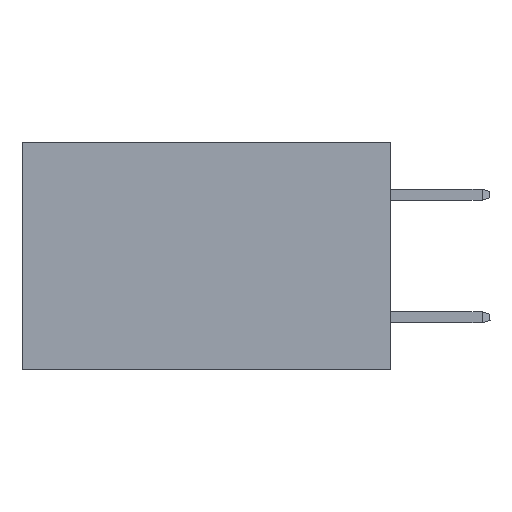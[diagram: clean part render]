
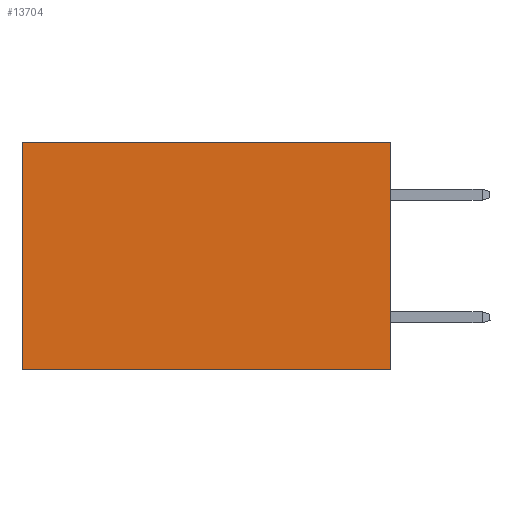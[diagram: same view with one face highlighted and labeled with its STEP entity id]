
A CAD part, left-side view. The second image highlights one B-rep face of the part: STEP entity #13704.
In plain terms, the highlighted planar face has unit normal (-1, 0, 0).
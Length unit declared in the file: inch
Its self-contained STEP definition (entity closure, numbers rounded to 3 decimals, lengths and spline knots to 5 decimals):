
#299 = VECTOR ( 'NONE', #13434, 39.37008 ) ;
#579 = EDGE_CURVE ( 'NONE', #8888, #7208, #5115, .T. ) ;
#962 = LINE ( 'NONE', #8268, #7825 ) ;
#1601 = VECTOR ( 'NONE', #4179, 39.37008 ) ;
#1996 = LINE ( 'NONE', #9950, #7703 ) ;
#2992 = VERTEX_POINT ( 'NONE', #15432 ) ;
#3164 = CARTESIAN_POINT ( 'NONE',  ( 0.2875, 0., 0. ) ) ;
#3614 = EDGE_CURVE ( 'NONE', #6200, #2992, #15764, .T. ) ;
#3931 = DIRECTION ( 'NONE',  ( 1., 0., 0. ) ) ;
#4169 = ORIENTED_EDGE ( 'NONE', *, *, #579, .F. ) ;
#4179 = DIRECTION ( 'NONE',  ( 0., 1., 0. ) ) ;
#4520 = CARTESIAN_POINT ( 'NONE',  ( 0.2875, 0.6, -0.37 ) ) ;
#4759 = DIRECTION ( 'NONE',  ( 0., 0., -1. ) ) ;
#4947 = DIRECTION ( 'NONE',  ( 0., 0., -1. ) ) ;
#5115 = LINE ( 'NONE', #10947, #299 ) ;
#6200 = VERTEX_POINT ( 'NONE', #3164 ) ;
#7086 = FACE_OUTER_BOUND ( 'NONE', #13526, .T. ) ;
#7208 = VERTEX_POINT ( 'NONE', #4520 ) ;
#7384 = PLANE ( 'NONE',  #14642 ) ;
#7703 = VECTOR ( 'NONE', #4947, 39.37008 ) ;
#7825 = VECTOR ( 'NONE', #4759, 39.37008 ) ;
#8202 = ORIENTED_EDGE ( 'NONE', *, *, #3614, .T. ) ;
#8268 = CARTESIAN_POINT ( 'NONE',  ( 0.2875, 0., 0. ) ) ;
#8604 = CARTESIAN_POINT ( 'NONE',  ( 0.2875, 0., 0. ) ) ;
#8888 = VERTEX_POINT ( 'NONE', #12912 ) ;
#9950 = CARTESIAN_POINT ( 'NONE',  ( 0.2875, 0.6, 0. ) ) ;
#10947 = CARTESIAN_POINT ( 'NONE',  ( 0.2875, 0., -0.37 ) ) ;
#11512 = CARTESIAN_POINT ( 'NONE',  ( 0.2875, 0., 0. ) ) ;
#12360 = EDGE_CURVE ( 'NONE', #2992, #7208, #1996, .T. ) ;
#12912 = CARTESIAN_POINT ( 'NONE',  ( 0.2875, 0., -0.37 ) ) ;
#13434 = DIRECTION ( 'NONE',  ( 0., 1., 0. ) ) ;
#13526 = EDGE_LOOP ( 'NONE', ( #14466, #4169, #13948, #8202 ) ) ;
#13704 = ADVANCED_FACE ( 'NONE', ( #7086 ), #7384, .F. ) ;
#13746 = DIRECTION ( 'NONE',  ( 0., 0., -1. ) ) ;
#13948 = ORIENTED_EDGE ( 'NONE', *, *, #13987, .F. ) ;
#13987 = EDGE_CURVE ( 'NONE', #6200, #8888, #962, .T. ) ;
#14466 = ORIENTED_EDGE ( 'NONE', *, *, #12360, .T. ) ;
#14642 = AXIS2_PLACEMENT_3D ( 'NONE', #8604, #3931, #13746 ) ;
#15432 = CARTESIAN_POINT ( 'NONE',  ( 0.2875, 0.6, 0. ) ) ;
#15764 = LINE ( 'NONE', #11512, #1601 ) ;
